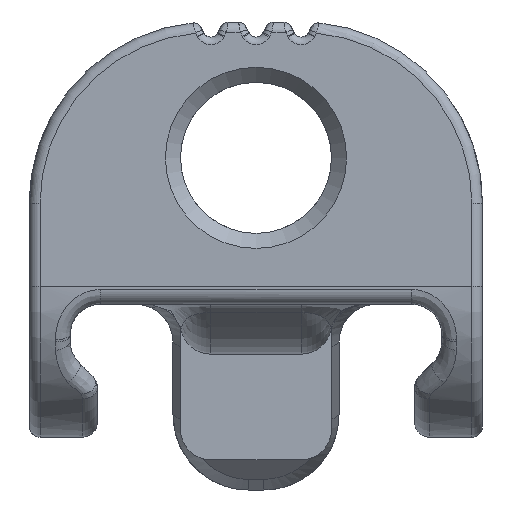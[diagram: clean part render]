
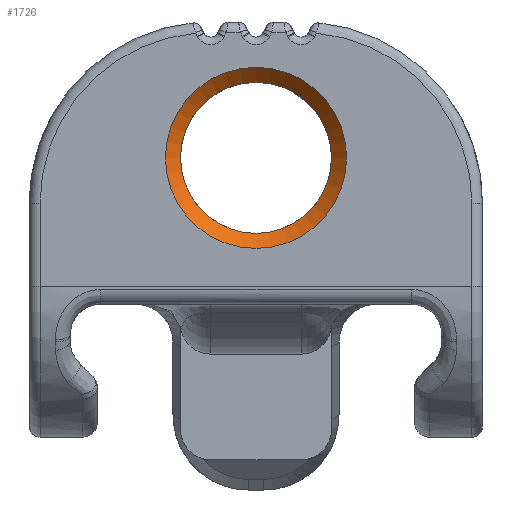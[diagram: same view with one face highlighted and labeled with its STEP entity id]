
A CAD part, left-side view. The second image highlights one B-rep face of the part: STEP entity #1726.
In plain terms, the highlighted conical face has half-angle 45 degrees and reference radius 5 mm.
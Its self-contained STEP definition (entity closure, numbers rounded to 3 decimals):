
#22 = VERTEX_POINT('',#23);
#23 = CARTESIAN_POINT('',(1.,0.,-5.));
#32 = CYLINDRICAL_SURFACE('',#33,5.);
#33 = AXIS2_PLACEMENT_3D('',#34,#35,#36);
#34 = CARTESIAN_POINT('',(-6.,0.,0.));
#35 = DIRECTION('',(-1.,-0.,0.));
#36 = DIRECTION('',(0.,0.,-1.));
#1594 = EDGE_CURVE('',#22,#22,#1595,.T.);
#1595 = SURFACE_CURVE('',#1596,(#1601,#1608),.PCURVE_S1.);
#1596 = CIRCLE('',#1597,5.);
#1597 = AXIS2_PLACEMENT_3D('',#1598,#1599,#1600);
#1598 = CARTESIAN_POINT('',(1.,0.,0.));
#1599 = DIRECTION('',(-1.,-0.,-0.));
#1600 = DIRECTION('',(0.,0.,-1.));
#1601 = PCURVE('',#32,#1602);
#1602 = DEFINITIONAL_REPRESENTATION('',(#1603),#1607);
#1603 = LINE('',#1604,#1605);
#1604 = CARTESIAN_POINT('',(-6.283,-7.));
#1605 = VECTOR('',#1606,1.);
#1606 = DIRECTION('',(1.,-0.));
#1607 = ( GEOMETRIC_REPRESENTATION_CONTEXT(2) 
PARAMETRIC_REPRESENTATION_CONTEXT() REPRESENTATION_CONTEXT('2D SPACE',''
  ) );
#1608 = PCURVE('',#1609,#1614);
#1609 = CONICAL_SURFACE('',#1610,5.,0.785);
#1610 = AXIS2_PLACEMENT_3D('',#1611,#1612,#1613);
#1611 = CARTESIAN_POINT('',(1.,0.,0.));
#1612 = DIRECTION('',(-1.,0.,0.));
#1613 = DIRECTION('',(0.,0.,-1.));
#1614 = DEFINITIONAL_REPRESENTATION('',(#1615),#1619);
#1615 = LINE('',#1616,#1617);
#1616 = CARTESIAN_POINT('',(0.,-0.));
#1617 = VECTOR('',#1618,1.);
#1618 = DIRECTION('',(1.,-0.));
#1619 = ( GEOMETRIC_REPRESENTATION_CONTEXT(2) 
PARAMETRIC_REPRESENTATION_CONTEXT() REPRESENTATION_CONTEXT('2D SPACE',''
  ) );
#1726 = ADVANCED_FACE('',(#1727),#1609,.F.);
#1727 = FACE_BOUND('',#1728,.T.);
#1728 = EDGE_LOOP('',(#1729,#1750,#1781,#1782));
#1729 = ORIENTED_EDGE('',*,*,#1730,.F.);
#1730 = EDGE_CURVE('',#1731,#22,#1733,.T.);
#1731 = VERTEX_POINT('',#1732);
#1732 = CARTESIAN_POINT('',(0.,0.,-6.));
#1733 = SEAM_CURVE('',#1734,(#1738,#1744),.PCURVE_S1.);
#1734 = LINE('',#1735,#1736);
#1735 = CARTESIAN_POINT('',(1.,0.,-5.));
#1736 = VECTOR('',#1737,1.);
#1737 = DIRECTION('',(0.707,0.,0.707));
#1738 = PCURVE('',#1609,#1739);
#1739 = DEFINITIONAL_REPRESENTATION('',(#1740),#1743);
#1740 = B_SPLINE_CURVE_WITH_KNOTS('',1,(#1741,#1742),.UNSPECIFIED.,.F.,
  .F.,(2,2),(-1.414,0.),.PIECEWISE_BEZIER_KNOTS.);
#1741 = CARTESIAN_POINT('',(0.,1.));
#1742 = CARTESIAN_POINT('',(0.,0.));
#1743 = ( GEOMETRIC_REPRESENTATION_CONTEXT(2) 
PARAMETRIC_REPRESENTATION_CONTEXT() REPRESENTATION_CONTEXT('2D SPACE',''
  ) );
#1744 = PCURVE('',#1609,#1745);
#1745 = DEFINITIONAL_REPRESENTATION('',(#1746),#1749);
#1746 = B_SPLINE_CURVE_WITH_KNOTS('',1,(#1747,#1748),.UNSPECIFIED.,.F.,
  .F.,(2,2),(-1.414,0.),.PIECEWISE_BEZIER_KNOTS.);
#1747 = CARTESIAN_POINT('',(6.283,1.));
#1748 = CARTESIAN_POINT('',(6.283,0.));
#1749 = ( GEOMETRIC_REPRESENTATION_CONTEXT(2) 
PARAMETRIC_REPRESENTATION_CONTEXT() REPRESENTATION_CONTEXT('2D SPACE',''
  ) );
#1750 = ORIENTED_EDGE('',*,*,#1751,.T.);
#1751 = EDGE_CURVE('',#1731,#1731,#1752,.T.);
#1752 = SURFACE_CURVE('',#1753,(#1758,#1765),.PCURVE_S1.);
#1753 = CIRCLE('',#1754,6.);
#1754 = AXIS2_PLACEMENT_3D('',#1755,#1756,#1757);
#1755 = CARTESIAN_POINT('',(0.,0.,0.));
#1756 = DIRECTION('',(-1.,-0.,-0.));
#1757 = DIRECTION('',(0.,0.,-1.));
#1758 = PCURVE('',#1609,#1759);
#1759 = DEFINITIONAL_REPRESENTATION('',(#1760),#1764);
#1760 = LINE('',#1761,#1762);
#1761 = CARTESIAN_POINT('',(-0.,1.));
#1762 = VECTOR('',#1763,1.);
#1763 = DIRECTION('',(1.,-0.));
#1764 = ( GEOMETRIC_REPRESENTATION_CONTEXT(2) 
PARAMETRIC_REPRESENTATION_CONTEXT() REPRESENTATION_CONTEXT('2D SPACE',''
  ) );
#1765 = PCURVE('',#1766,#1771);
#1766 = PLANE('',#1767);
#1767 = AXIS2_PLACEMENT_3D('',#1768,#1769,#1770);
#1768 = CARTESIAN_POINT('',(0.,-15.,-18.5));
#1769 = DIRECTION('',(1.,0.,0.));
#1770 = DIRECTION('',(0.,0.,1.));
#1771 = DEFINITIONAL_REPRESENTATION('',(#1772),#1780);
#1772 = ( BOUNDED_CURVE() B_SPLINE_CURVE(2,(#1773,#1774,#1775,#1776,
#1777,#1778,#1779),.UNSPECIFIED.,.T.,.F.) B_SPLINE_CURVE_WITH_KNOTS((1,2
    ,2,2,2,1),(-2.094,0.,2.094,4.189,
6.283,8.378),.UNSPECIFIED.) CURVE() 
GEOMETRIC_REPRESENTATION_ITEM() RATIONAL_B_SPLINE_CURVE((1.,0.5,1.,0.5,
1.,0.5,1.)) REPRESENTATION_ITEM('') );
#1773 = CARTESIAN_POINT('',(12.5,-15.));
#1774 = CARTESIAN_POINT('',(12.5,-4.608));
#1775 = CARTESIAN_POINT('',(21.5,-9.804));
#1776 = CARTESIAN_POINT('',(30.5,-15.));
#1777 = CARTESIAN_POINT('',(21.5,-20.196));
#1778 = CARTESIAN_POINT('',(12.5,-25.392));
#1779 = CARTESIAN_POINT('',(12.5,-15.));
#1780 = ( GEOMETRIC_REPRESENTATION_CONTEXT(2) 
PARAMETRIC_REPRESENTATION_CONTEXT() REPRESENTATION_CONTEXT('2D SPACE',''
  ) );
#1781 = ORIENTED_EDGE('',*,*,#1730,.T.);
#1782 = ORIENTED_EDGE('',*,*,#1594,.F.);
